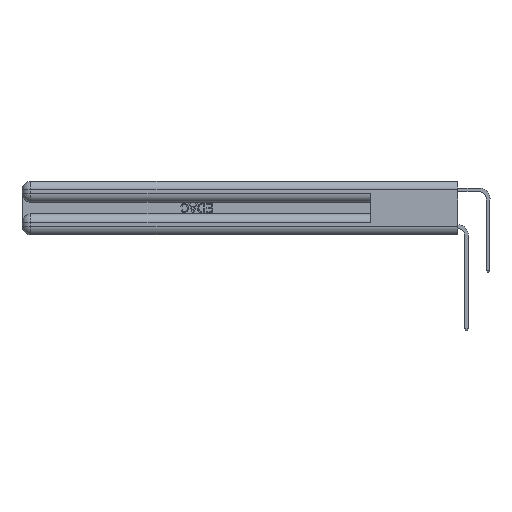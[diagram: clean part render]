
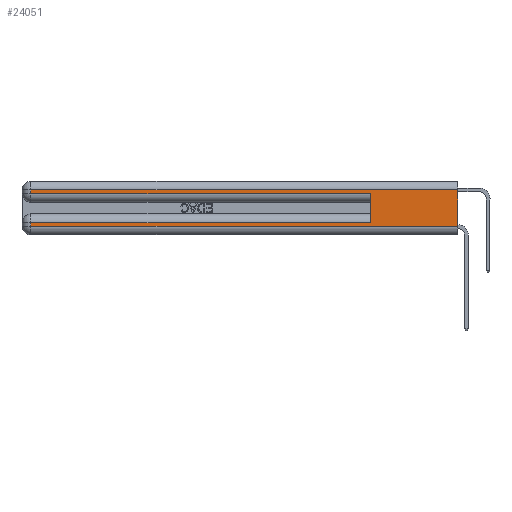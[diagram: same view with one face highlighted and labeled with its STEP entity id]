
A CAD part, left-side view. The second image highlights one B-rep face of the part: STEP entity #24051.
In plain terms, the highlighted planar face has unit normal (-1, 0, 0).
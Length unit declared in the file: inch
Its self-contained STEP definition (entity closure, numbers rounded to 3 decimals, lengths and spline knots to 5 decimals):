
#105 = ORIENTED_EDGE ( 'NONE', *, *, #5933, .T. ) ;
#236 = CARTESIAN_POINT ( 'NONE',  ( 0., 0.6, 0.145 ) ) ;
#594 = LINE ( 'NONE', #3097, #17127 ) ;
#636 = ORIENTED_EDGE ( 'NONE', *, *, #18961, .T. ) ;
#1341 = ORIENTED_EDGE ( 'NONE', *, *, #17669, .T. ) ;
#1409 = CARTESIAN_POINT ( 'NONE',  ( 0., 2.94, 0.37 ) ) ;
#1988 = DIRECTION ( 'NONE',  ( 0., 1., 0. ) ) ;
#3097 = CARTESIAN_POINT ( 'NONE',  ( 0., 0., 0.06 ) ) ;
#3225 = VECTOR ( 'NONE', #6123, 39.37008 ) ;
#4264 = CARTESIAN_POINT ( 'NONE',  ( 0., 2.94, 0.37 ) ) ;
#4780 = EDGE_LOOP ( 'NONE', ( #15509, #24496, #1341, #105, #16444, #11938, #636, #8453 ) ) ;
#5267 = DIRECTION ( 'NONE',  ( 0., 0., -1. ) ) ;
#5315 = VECTOR ( 'NONE', #15003, 39.37008 ) ;
#5933 = EDGE_CURVE ( 'NONE', #11905, #15899, #9044, .T. ) ;
#6123 = DIRECTION ( 'NONE',  ( 0., 0., -1. ) ) ;
#6445 = VECTOR ( 'NONE', #1988, 39.37008 ) ;
#7620 = CARTESIAN_POINT ( 'NONE',  ( 0., 2.94, 0.31 ) ) ;
#8149 = EDGE_CURVE ( 'NONE', #20995, #9354, #594, .T. ) ;
#8175 = DIRECTION ( 'NONE',  ( 0., 0., -1. ) ) ;
#8453 = ORIENTED_EDGE ( 'NONE', *, *, #8149, .T. ) ;
#9044 = LINE ( 'NONE', #10750, #17722 ) ;
#9354 = VERTEX_POINT ( 'NONE', #25186 ) ;
#10078 = CARTESIAN_POINT ( 'NONE',  ( 0., 0.6, 0.085 ) ) ;
#10712 = DIRECTION ( 'NONE',  ( 0., 1., 0. ) ) ;
#10750 = CARTESIAN_POINT ( 'NONE',  ( 0., 0., 0.285 ) ) ;
#11905 = VERTEX_POINT ( 'NONE', #19144 ) ;
#11938 = ORIENTED_EDGE ( 'NONE', *, *, #12422, .T. ) ;
#11957 = PLANE ( 'NONE',  #13589 ) ;
#12258 = LINE ( 'NONE', #1409, #3225 ) ;
#12422 = EDGE_CURVE ( 'NONE', #23016, #22984, #27382, .T. ) ;
#13410 = DIRECTION ( 'NONE',  ( 0., -1., 0. ) ) ;
#13589 = AXIS2_PLACEMENT_3D ( 'NONE', #22408, #20043, #5267 ) ;
#13727 = CARTESIAN_POINT ( 'NONE',  ( 0., 2.94, 0.085 ) ) ;
#14088 = EDGE_CURVE ( 'NONE', #24220, #9354, #18674, .T. ) ;
#14170 = FACE_OUTER_BOUND ( 'NONE', #4780, .T. ) ;
#14466 = VECTOR ( 'NONE', #10712, 39.37008 ) ;
#14729 = CARTESIAN_POINT ( 'NONE',  ( 0., 0., 0.31 ) ) ;
#14740 = EDGE_CURVE ( 'NONE', #23016, #15899, #19054, .T. ) ;
#15003 = DIRECTION ( 'NONE',  ( 0., 0., 1. ) ) ;
#15509 = ORIENTED_EDGE ( 'NONE', *, *, #14088, .F. ) ;
#15899 = VERTEX_POINT ( 'NONE', #27192 ) ;
#16444 = ORIENTED_EDGE ( 'NONE', *, *, #14740, .F. ) ;
#16653 = VECTOR ( 'NONE', #8175, 39.37008 ) ;
#17127 = VECTOR ( 'NONE', #13410, 39.37008 ) ;
#17669 = EDGE_CURVE ( 'NONE', #22691, #11905, #27311, .T. ) ;
#17722 = VECTOR ( 'NONE', #26087, 39.37008 ) ;
#18674 = LINE ( 'NONE', #27218, #27566 ) ;
#18805 = DIRECTION ( 'NONE',  ( 0., 0., -1. ) ) ;
#18961 = EDGE_CURVE ( 'NONE', #22984, #20995, #12258, .T. ) ;
#19054 = LINE ( 'NONE', #236, #5315 ) ;
#19116 = CARTESIAN_POINT ( 'NONE',  ( 0., 0., 0.085 ) ) ;
#19144 = CARTESIAN_POINT ( 'NONE',  ( 0., 2.94, 0.285 ) ) ;
#20043 = DIRECTION ( 'NONE',  ( 1., 0., 0. ) ) ;
#20995 = VERTEX_POINT ( 'NONE', #22252 ) ;
#21299 = CARTESIAN_POINT ( 'NONE',  ( 0., 0., 0.31 ) ) ;
#21708 = LINE ( 'NONE', #21299, #14466 ) ;
#22252 = CARTESIAN_POINT ( 'NONE',  ( 0., 2.94, 0.06 ) ) ;
#22408 = CARTESIAN_POINT ( 'NONE',  ( 0., 0., 0.37 ) ) ;
#22691 = VERTEX_POINT ( 'NONE', #7620 ) ;
#22984 = VERTEX_POINT ( 'NONE', #13727 ) ;
#23016 = VERTEX_POINT ( 'NONE', #10078 ) ;
#24051 = ADVANCED_FACE ( 'NONE', ( #14170 ), #11957, .F. ) ;
#24220 = VERTEX_POINT ( 'NONE', #14729 ) ;
#24369 = EDGE_CURVE ( 'NONE', #24220, #22691, #21708, .T. ) ;
#24496 = ORIENTED_EDGE ( 'NONE', *, *, #24369, .T. ) ;
#25186 = CARTESIAN_POINT ( 'NONE',  ( 0., 0., 0.06 ) ) ;
#26087 = DIRECTION ( 'NONE',  ( 0., -1., 0. ) ) ;
#27192 = CARTESIAN_POINT ( 'NONE',  ( 0., 0.6, 0.285 ) ) ;
#27218 = CARTESIAN_POINT ( 'NONE',  ( 0., 0., 0.37 ) ) ;
#27311 = LINE ( 'NONE', #4264, #16653 ) ;
#27382 = LINE ( 'NONE', #19116, #6445 ) ;
#27566 = VECTOR ( 'NONE', #18805, 39.37008 ) ;
